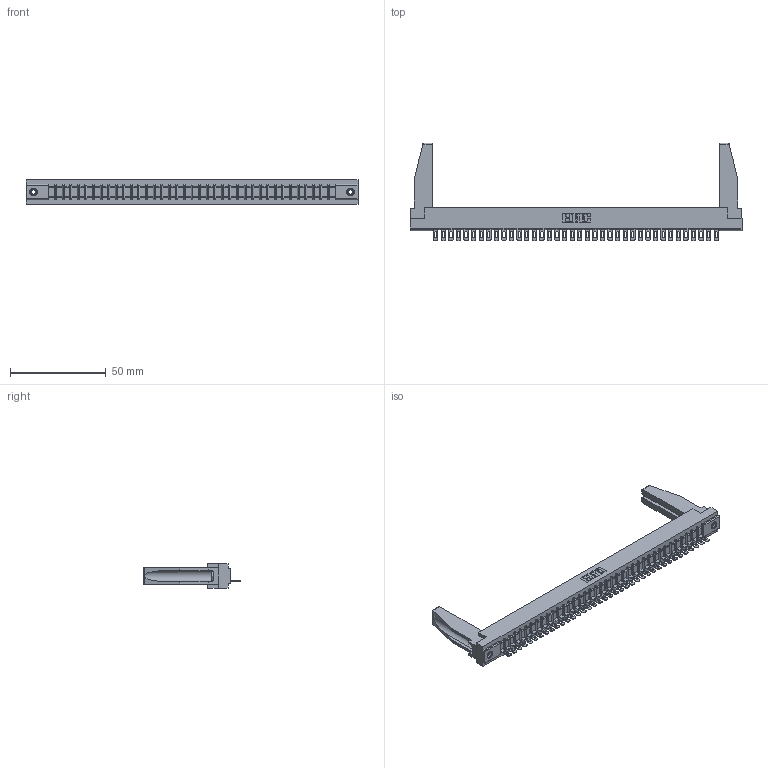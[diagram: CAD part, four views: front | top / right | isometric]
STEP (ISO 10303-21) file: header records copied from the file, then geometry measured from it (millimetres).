
FILE_DESCRIPTION (( 'STEP AP203' ), '1' );
FILE_NAME ('357-038-501-178.STEP', '2019-09-17T07:38:55', ( '' ), ( '' ), 'SwSTEP 2.0', 'SolidWorks 2016', '' );
FILE_SCHEMA (( 'CONFIG_CONTROL_DESIGN' ));
Length unit declared in the file: inch
Products named in the file (5): 307-290-002_501; 307-220-078; 307 Part_.156 Dia Mounting Holes; 357-038-501-178; 345-250-001_345-250-001-102
Assembly tree (43 placements, depth 2):
  357-038-501-178
    307 Part_.156 Dia Mounting Holes
    307-290-002_501  x38
    307-220-078  x2
    345-250-001_345-250-001-102  x2
Bounding box: 173.58 x 51.13 x 12.7 mm (x, y, z)
Volume: 22572.2 mm3; surface area: 27354.7 mm2
Topology: 43 solids, 43 shells, 3175 faces, 9697 edges, 6350 vertices
Faces by surface type: plane 1826, cylinder 1255, sphere 78, cone 12, torus 4
Entity records: 36303 total; most frequent: CARTESIAN_POINT 6122, ORIENTED_EDGE 6068, DIRECTION 5910, EDGE_CURVE 3034, VECTOR 2322, LINE 2322, VERTEX_POINT 1964, AXIS2_PLACEMENT_3D 1794
